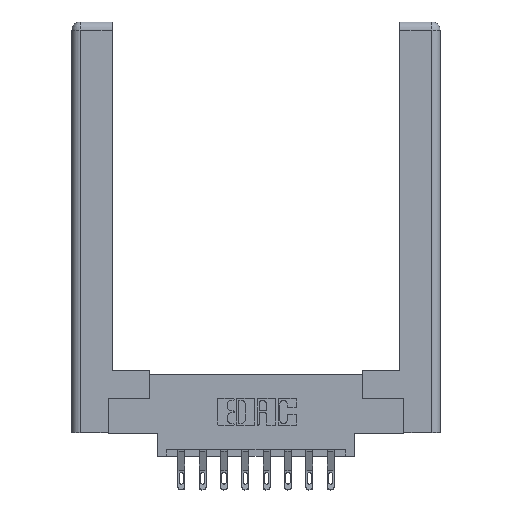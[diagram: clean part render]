
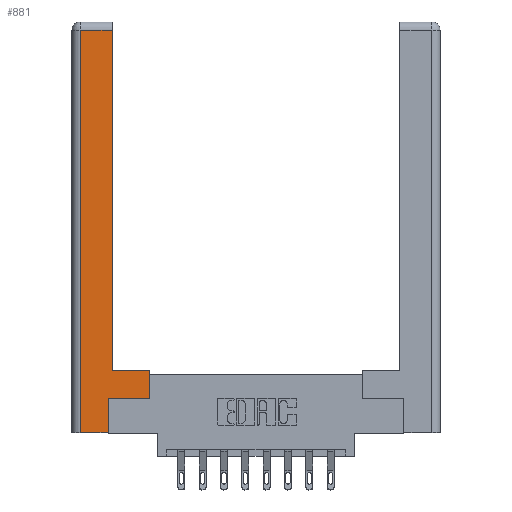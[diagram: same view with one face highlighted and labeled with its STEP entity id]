
A CAD part, top view. The second image highlights one B-rep face of the part: STEP entity #881.
In plain terms, the highlighted planar face has unit normal (0, 0, 1).
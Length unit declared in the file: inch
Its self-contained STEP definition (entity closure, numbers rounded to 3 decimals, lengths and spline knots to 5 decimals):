
#54 = CARTESIAN_POINT ( 'NONE',  ( 0.565, 0.45, 0. ) ) ;
#239 = DIRECTION ( 'NONE',  ( 0., 1., 0. ) ) ;
#265 = CARTESIAN_POINT ( 'NONE',  ( 0., 0., 0. ) ) ;
#322 = DIRECTION ( 'NONE',  ( -1., 0., 0. ) ) ;
#372 = CARTESIAN_POINT ( 'NONE',  ( 0.0615, 0., 0. ) ) ;
#817 = LINE ( 'NONE', #9638, #8625 ) ;
#881 = ADVANCED_FACE ( 'NONE', ( #950 ), #2382, .F. ) ;
#950 = FACE_OUTER_BOUND ( 'NONE', #5371, .T. ) ;
#1187 = LINE ( 'NONE', #2929, #8639 ) ;
#1231 = ORIENTED_EDGE ( 'NONE', *, *, #3484, .T. ) ;
#1413 = VECTOR ( 'NONE', #322, 39.37008 ) ;
#1566 = DIRECTION ( 'NONE',  ( -1., 0., 0. ) ) ;
#1798 = DIRECTION ( 'NONE',  ( 1., 0., 0. ) ) ;
#2309 = EDGE_CURVE ( 'NONE', #5937, #8517, #11011, .T. ) ;
#2356 = VECTOR ( 'NONE', #1566, 39.37008 ) ;
#2382 = PLANE ( 'NONE',  #13582 ) ;
#2607 = CARTESIAN_POINT ( 'NONE',  ( 0.0615, 2.94, 0. ) ) ;
#2929 = CARTESIAN_POINT ( 'NONE',  ( 0.265, 0., 0. ) ) ;
#3092 = ORIENTED_EDGE ( 'NONE', *, *, #6460, .T. ) ;
#3134 = VERTEX_POINT ( 'NONE', #13012 ) ;
#3264 = CARTESIAN_POINT ( 'NONE',  ( 0.565, 0.245, 0. ) ) ;
#3484 = EDGE_CURVE ( 'NONE', #7358, #5937, #3726, .T. ) ;
#3552 = DIRECTION ( 'NONE',  ( -1., 0., 0. ) ) ;
#3629 = VERTEX_POINT ( 'NONE', #7289 ) ;
#3726 = LINE ( 'NONE', #11292, #6005 ) ;
#3777 = CARTESIAN_POINT ( 'NONE',  ( 0.565, 0.245, 0. ) ) ;
#4018 = LINE ( 'NONE', #3264, #7817 ) ;
#4349 = EDGE_CURVE ( 'NONE', #8517, #3134, #10300, .T. ) ;
#4665 = LINE ( 'NONE', #7988, #12415 ) ;
#4895 = ORIENTED_EDGE ( 'NONE', *, *, #13382, .T. ) ;
#4997 = LINE ( 'NONE', #2607, #2356 ) ;
#5334 = EDGE_CURVE ( 'NONE', #7221, #7358, #4018, .T. ) ;
#5371 = EDGE_LOOP ( 'NONE', ( #8783, #10800, #13606, #3092, #4895, #6050, #1231, #8174 ) ) ;
#5937 = VERTEX_POINT ( 'NONE', #54 ) ;
#6005 = VECTOR ( 'NONE', #6014, 39.37008 ) ;
#6014 = DIRECTION ( 'NONE',  ( 0., 1., 0. ) ) ;
#6050 = ORIENTED_EDGE ( 'NONE', *, *, #5334, .T. ) ;
#6350 = EDGE_CURVE ( 'NONE', #3134, #3629, #4997, .T. ) ;
#6460 = EDGE_CURVE ( 'NONE', #11825, #10034, #1187, .T. ) ;
#7221 = VERTEX_POINT ( 'NONE', #7783 ) ;
#7289 = CARTESIAN_POINT ( 'NONE',  ( 0.0615, 2.94, 0. ) ) ;
#7358 = VERTEX_POINT ( 'NONE', #3777 ) ;
#7421 = EDGE_CURVE ( 'NONE', #3629, #11825, #4665, .T. ) ;
#7474 = DIRECTION ( 'NONE',  ( 1., 0., 0. ) ) ;
#7691 = VECTOR ( 'NONE', #239, 39.37008 ) ;
#7783 = CARTESIAN_POINT ( 'NONE',  ( 0.265, 0.245, 0. ) ) ;
#7817 = VECTOR ( 'NONE', #7474, 39.37008 ) ;
#7988 = CARTESIAN_POINT ( 'NONE',  ( 0.0615, 0., 0. ) ) ;
#8174 = ORIENTED_EDGE ( 'NONE', *, *, #2309, .T. ) ;
#8517 = VERTEX_POINT ( 'NONE', #10355 ) ;
#8625 = VECTOR ( 'NONE', #10317, 39.37008 ) ;
#8639 = VECTOR ( 'NONE', #1798, 39.37008 ) ;
#8783 = ORIENTED_EDGE ( 'NONE', *, *, #4349, .T. ) ;
#8921 = CARTESIAN_POINT ( 'NONE',  ( 0.295, 0.45, 0. ) ) ;
#8937 = CARTESIAN_POINT ( 'NONE',  ( 0.295, 3., 0. ) ) ;
#8956 = DIRECTION ( 'NONE',  ( 0., -1., 0. ) ) ;
#9638 = CARTESIAN_POINT ( 'NONE',  ( 0.265, 0.245, 0. ) ) ;
#9815 = DIRECTION ( 'NONE',  ( 0., 0., -1. ) ) ;
#10034 = VERTEX_POINT ( 'NONE', #10518 ) ;
#10300 = LINE ( 'NONE', #8937, #7691 ) ;
#10317 = DIRECTION ( 'NONE',  ( 0., 1., 0. ) ) ;
#10355 = CARTESIAN_POINT ( 'NONE',  ( 0.295, 0.45, 0. ) ) ;
#10518 = CARTESIAN_POINT ( 'NONE',  ( 0.265, 0., 0. ) ) ;
#10800 = ORIENTED_EDGE ( 'NONE', *, *, #6350, .T. ) ;
#11011 = LINE ( 'NONE', #8921, #1413 ) ;
#11292 = CARTESIAN_POINT ( 'NONE',  ( 0.565, 0.45, 0. ) ) ;
#11825 = VERTEX_POINT ( 'NONE', #372 ) ;
#12415 = VECTOR ( 'NONE', #8956, 39.37008 ) ;
#13012 = CARTESIAN_POINT ( 'NONE',  ( 0.295, 2.94, 0. ) ) ;
#13382 = EDGE_CURVE ( 'NONE', #10034, #7221, #817, .T. ) ;
#13582 = AXIS2_PLACEMENT_3D ( 'NONE', #265, #9815, #3552 ) ;
#13606 = ORIENTED_EDGE ( 'NONE', *, *, #7421, .T. ) ;
